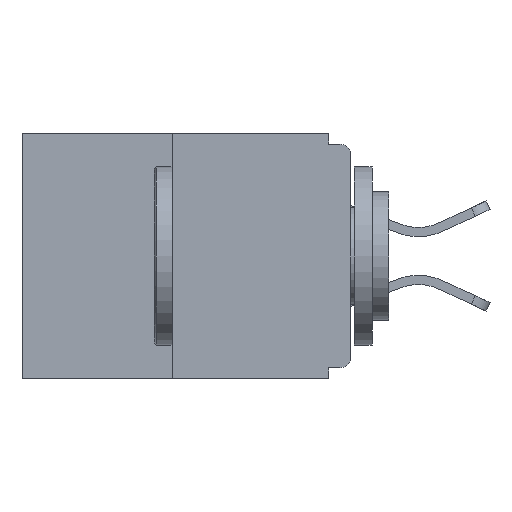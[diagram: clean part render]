
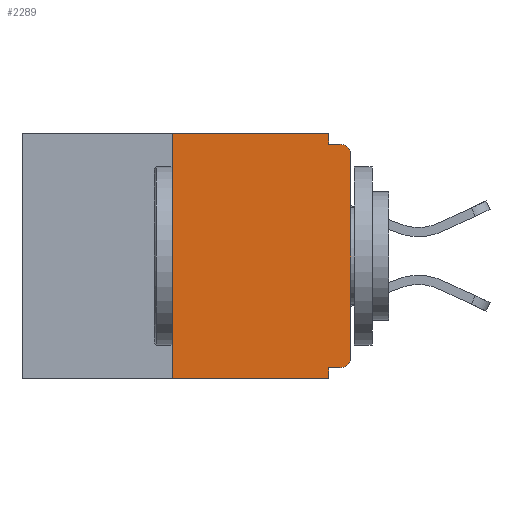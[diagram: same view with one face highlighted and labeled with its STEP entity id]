
A CAD part, left-side view. The second image highlights one B-rep face of the part: STEP entity #2289.
In plain terms, the highlighted planar face has unit normal (-1, 0, 0).
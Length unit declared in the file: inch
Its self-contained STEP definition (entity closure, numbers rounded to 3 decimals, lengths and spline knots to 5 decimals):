
#565 = CARTESIAN_POINT ( 'NONE',  ( 0., 0., -0.328 ) ) ;
#685 = DIRECTION ( 'NONE',  ( 0., 0., 1. ) ) ;
#745 = CARTESIAN_POINT ( 'NONE',  ( 0., 0.015, -0.03 ) ) ;
#763 = LINE ( 'NONE', #565, #9145 ) ;
#801 = EDGE_CURVE ( 'NONE', #8768, #6499, #10909, .T. ) ;
#817 = CARTESIAN_POINT ( 'NONE',  ( 0., 0., -0.03 ) ) ;
#1004 = CARTESIAN_POINT ( 'NONE',  ( 0., 0.25, 0. ) ) ;
#1008 = CARTESIAN_POINT ( 'NONE',  ( 0., 0., -0.313 ) ) ;
#1061 = EDGE_CURVE ( 'NONE', #1849, #11006, #4577, .T. ) ;
#1193 = DIRECTION ( 'NONE',  ( 0., 0., 1. ) ) ;
#1674 = AXIS2_PLACEMENT_3D ( 'NONE', #3216, #11613, #2321 ) ;
#1727 = EDGE_CURVE ( 'NONE', #9516, #11094, #2090, .T. ) ;
#1733 = CARTESIAN_POINT ( 'NONE',  ( 0., 0.46, -0.343 ) ) ;
#1849 = VERTEX_POINT ( 'NONE', #11060 ) ;
#1858 = DIRECTION ( 'NONE',  ( -1., 0., 0. ) ) ;
#2090 = LINE ( 'NONE', #1733, #5894 ) ;
#2289 = ADVANCED_FACE ( 'NONE', ( #3247 ), #11517, .F. ) ;
#2321 = DIRECTION ( 'NONE',  ( 0., 0., -1. ) ) ;
#2542 = DIRECTION ( 'NONE',  ( 0., -1., 0. ) ) ;
#3188 = LINE ( 'NONE', #12098, #4642 ) ;
#3216 = CARTESIAN_POINT ( 'NONE',  ( 0., 0.46, 0. ) ) ;
#3247 = FACE_OUTER_BOUND ( 'NONE', #7924, .T. ) ;
#3387 = DIRECTION ( 'NONE',  ( 0., -1., 0. ) ) ;
#3716 = DIRECTION ( 'NONE',  ( 0., 0., -1. ) ) ;
#3858 = ORIENTED_EDGE ( 'NONE', *, *, #1061, .F. ) ;
#3988 = CARTESIAN_POINT ( 'NONE',  ( 0., 0.015, -0.328 ) ) ;
#4114 = CARTESIAN_POINT ( 'NONE',  ( 0., 0.25, -0.343 ) ) ;
#4307 = AXIS2_PLACEMENT_3D ( 'NONE', #8474, #1858, #10176 ) ;
#4308 = VECTOR ( 'NONE', #1193, 39.37008 ) ;
#4332 = CARTESIAN_POINT ( 'NONE',  ( 0., 0.031, 0. ) ) ;
#4374 = EDGE_CURVE ( 'NONE', #6499, #7130, #11124, .T. ) ;
#4534 = VERTEX_POINT ( 'NONE', #8311 ) ;
#4577 = LINE ( 'NONE', #4332, #10760 ) ;
#4642 = VECTOR ( 'NONE', #7328, 39.37008 ) ;
#4726 = ORIENTED_EDGE ( 'NONE', *, *, #10513, .F. ) ;
#5034 = LINE ( 'NONE', #8051, #6672 ) ;
#5408 = VECTOR ( 'NONE', #11705, 39.37008 ) ;
#5768 = EDGE_CURVE ( 'NONE', #9516, #7034, #5034, .T. ) ;
#5852 = ORIENTED_EDGE ( 'NONE', *, *, #4374, .T. ) ;
#5894 = VECTOR ( 'NONE', #2542, 39.37008 ) ;
#5986 = VECTOR ( 'NONE', #3387, 39.37008 ) ;
#6289 = DIRECTION ( 'NONE',  ( -1., 0., 0. ) ) ;
#6309 = CIRCLE ( 'NONE', #4307, 0.015 ) ;
#6432 = EDGE_CURVE ( 'NONE', #11073, #4534, #763, .T. ) ;
#6499 = VERTEX_POINT ( 'NONE', #817 ) ;
#6672 = VECTOR ( 'NONE', #685, 39.37008 ) ;
#7012 = ORIENTED_EDGE ( 'NONE', *, *, #801, .T. ) ;
#7034 = VERTEX_POINT ( 'NONE', #1004 ) ;
#7085 = CARTESIAN_POINT ( 'NONE',  ( 0., 0., -0.015 ) ) ;
#7130 = VERTEX_POINT ( 'NONE', #9613 ) ;
#7220 = ORIENTED_EDGE ( 'NONE', *, *, #1727, .T. ) ;
#7328 = DIRECTION ( 'NONE',  ( 0., -1., 0. ) ) ;
#7924 = EDGE_LOOP ( 'NONE', ( #8421, #9950, #7220, #11758, #11473, #9300, #7012, #5852, #4726, #3858 ) ) ;
#7988 = EDGE_CURVE ( 'NONE', #11073, #8768, #6309, .T. ) ;
#8051 = CARTESIAN_POINT ( 'NONE',  ( 0., 0.25, 0. ) ) ;
#8268 = CARTESIAN_POINT ( 'NONE',  ( 0., 0.031, -0.343 ) ) ;
#8311 = CARTESIAN_POINT ( 'NONE',  ( 0., 0.031, -0.328 ) ) ;
#8421 = ORIENTED_EDGE ( 'NONE', *, *, #10185, .F. ) ;
#8444 = LINE ( 'NONE', #7085, #5986 ) ;
#8474 = CARTESIAN_POINT ( 'NONE',  ( 0., 0.015, -0.313 ) ) ;
#8768 = VERTEX_POINT ( 'NONE', #1008 ) ;
#9145 = VECTOR ( 'NONE', #10771, 39.37008 ) ;
#9300 = ORIENTED_EDGE ( 'NONE', *, *, #7988, .T. ) ;
#9302 = AXIS2_PLACEMENT_3D ( 'NONE', #745, #6289, #11881 ) ;
#9516 = VERTEX_POINT ( 'NONE', #4114 ) ;
#9613 = CARTESIAN_POINT ( 'NONE',  ( 0., 0.015, -0.015 ) ) ;
#9950 = ORIENTED_EDGE ( 'NONE', *, *, #5768, .F. ) ;
#9953 = LINE ( 'NONE', #10756, #5408 ) ;
#10176 = DIRECTION ( 'NONE',  ( 0., 0., -1. ) ) ;
#10185 = EDGE_CURVE ( 'NONE', #7034, #1849, #3188, .T. ) ;
#10513 = EDGE_CURVE ( 'NONE', #11006, #7130, #8444, .T. ) ;
#10543 = CARTESIAN_POINT ( 'NONE',  ( 0., 0., 0. ) ) ;
#10756 = CARTESIAN_POINT ( 'NONE',  ( 0., 0.031, -0.343 ) ) ;
#10760 = VECTOR ( 'NONE', #3716, 39.37008 ) ;
#10771 = DIRECTION ( 'NONE',  ( 0., 1., 0. ) ) ;
#10909 = LINE ( 'NONE', #10543, #4308 ) ;
#11006 = VERTEX_POINT ( 'NONE', #11533 ) ;
#11060 = CARTESIAN_POINT ( 'NONE',  ( 0., 0.031, 0. ) ) ;
#11073 = VERTEX_POINT ( 'NONE', #3988 ) ;
#11094 = VERTEX_POINT ( 'NONE', #8268 ) ;
#11124 = CIRCLE ( 'NONE', #9302, 0.015 ) ;
#11473 = ORIENTED_EDGE ( 'NONE', *, *, #6432, .F. ) ;
#11517 = PLANE ( 'NONE',  #1674 ) ;
#11523 = EDGE_CURVE ( 'NONE', #4534, #11094, #9953, .T. ) ;
#11533 = CARTESIAN_POINT ( 'NONE',  ( 0., 0.031, -0.015 ) ) ;
#11613 = DIRECTION ( 'NONE',  ( 1., 0., 0. ) ) ;
#11705 = DIRECTION ( 'NONE',  ( 0., 0., -1. ) ) ;
#11758 = ORIENTED_EDGE ( 'NONE', *, *, #11523, .F. ) ;
#11881 = DIRECTION ( 'NONE',  ( 0., 0., -1. ) ) ;
#12098 = CARTESIAN_POINT ( 'NONE',  ( 0., 0.46, 0. ) ) ;
